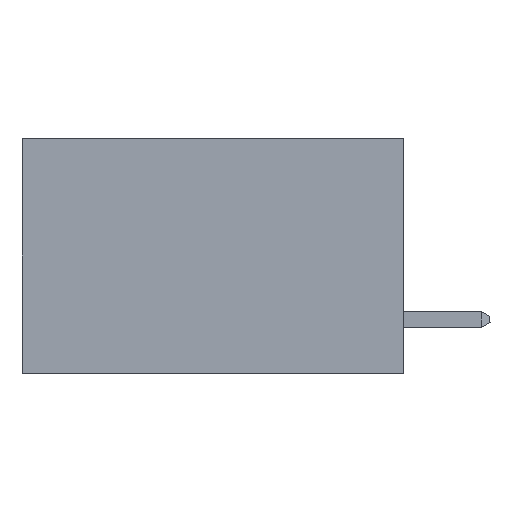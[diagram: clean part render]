
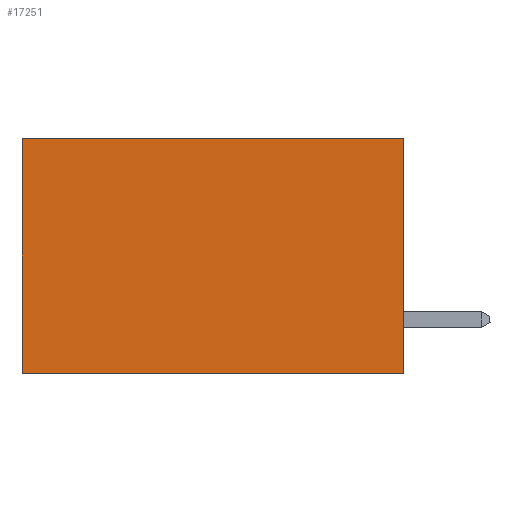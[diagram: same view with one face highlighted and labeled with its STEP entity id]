
A CAD part, left-side view. The second image highlights one B-rep face of the part: STEP entity #17251.
In plain terms, the highlighted planar face has unit normal (-1, 0, 0).
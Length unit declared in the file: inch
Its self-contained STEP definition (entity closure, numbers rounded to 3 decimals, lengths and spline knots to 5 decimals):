
#559 = ORIENTED_EDGE ( 'NONE', *, *, #12714, .T. ) ;
#1152 = LINE ( 'NONE', #19382, #33161 ) ;
#2725 = CARTESIAN_POINT ( 'NONE',  ( 0.2875, 0., 0. ) ) ;
#3293 = VECTOR ( 'NONE', #23297, 39.37008 ) ;
#3971 = DIRECTION ( 'NONE',  ( 0., 1., 0. ) ) ;
#4451 = ORIENTED_EDGE ( 'NONE', *, *, #30933, .T. ) ;
#5260 = LINE ( 'NONE', #8099, #3293 ) ;
#5864 = VERTEX_POINT ( 'NONE', #2725 ) ;
#6659 = CARTESIAN_POINT ( 'NONE',  ( 0.2875, 0., 0. ) ) ;
#7905 = VERTEX_POINT ( 'NONE', #8318 ) ;
#8008 = AXIS2_PLACEMENT_3D ( 'NONE', #26572, #32654, #36020 ) ;
#8099 = CARTESIAN_POINT ( 'NONE',  ( 0.2875, 0.6, 0. ) ) ;
#8318 = CARTESIAN_POINT ( 'NONE',  ( 0.2875, 0., -0.37 ) ) ;
#9459 = LINE ( 'NONE', #6659, #36627 ) ;
#10883 = VECTOR ( 'NONE', #19216, 39.37008 ) ;
#11946 = ORIENTED_EDGE ( 'NONE', *, *, #25442, .F. ) ;
#12591 = CARTESIAN_POINT ( 'NONE',  ( 0.2875, 0.6, 0. ) ) ;
#12714 = EDGE_CURVE ( 'NONE', #5864, #18294, #9459, .T. ) ;
#16634 = ORIENTED_EDGE ( 'NONE', *, *, #19461, .F. ) ;
#17251 = ADVANCED_FACE ( 'NONE', ( #29891 ), #29831, .F. ) ;
#18294 = VERTEX_POINT ( 'NONE', #12591 ) ;
#19216 = DIRECTION ( 'NONE',  ( 0., 0., -1. ) ) ;
#19382 = CARTESIAN_POINT ( 'NONE',  ( 0.2875, 0., -0.37 ) ) ;
#19461 = EDGE_CURVE ( 'NONE', #5864, #7905, #26419, .T. ) ;
#20332 = EDGE_LOOP ( 'NONE', ( #4451, #11946, #16634, #559 ) ) ;
#22701 = VERTEX_POINT ( 'NONE', #36007 ) ;
#23297 = DIRECTION ( 'NONE',  ( 0., 0., -1. ) ) ;
#25350 = CARTESIAN_POINT ( 'NONE',  ( 0.2875, 0., 0. ) ) ;
#25442 = EDGE_CURVE ( 'NONE', #7905, #22701, #1152, .T. ) ;
#26419 = LINE ( 'NONE', #25350, #10883 ) ;
#26572 = CARTESIAN_POINT ( 'NONE',  ( 0.2875, 0., 0. ) ) ;
#29831 = PLANE ( 'NONE',  #8008 ) ;
#29891 = FACE_OUTER_BOUND ( 'NONE', #20332, .T. ) ;
#30933 = EDGE_CURVE ( 'NONE', #18294, #22701, #5260, .T. ) ;
#31882 = DIRECTION ( 'NONE',  ( 0., 1., 0. ) ) ;
#32654 = DIRECTION ( 'NONE',  ( 1., 0., 0. ) ) ;
#33161 = VECTOR ( 'NONE', #3971, 39.37008 ) ;
#36007 = CARTESIAN_POINT ( 'NONE',  ( 0.2875, 0.6, -0.37 ) ) ;
#36020 = DIRECTION ( 'NONE',  ( 0., 0., -1. ) ) ;
#36627 = VECTOR ( 'NONE', #31882, 39.37008 ) ;
